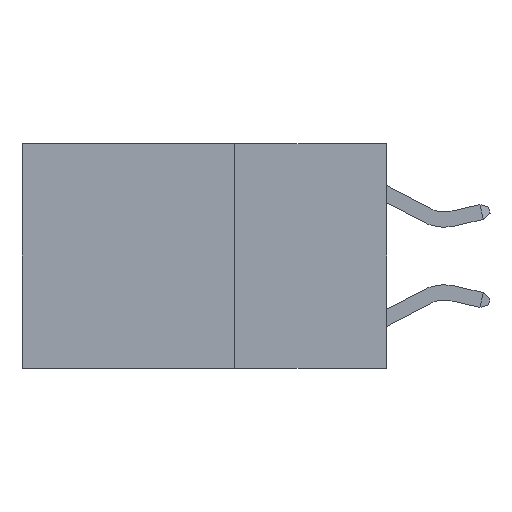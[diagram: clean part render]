
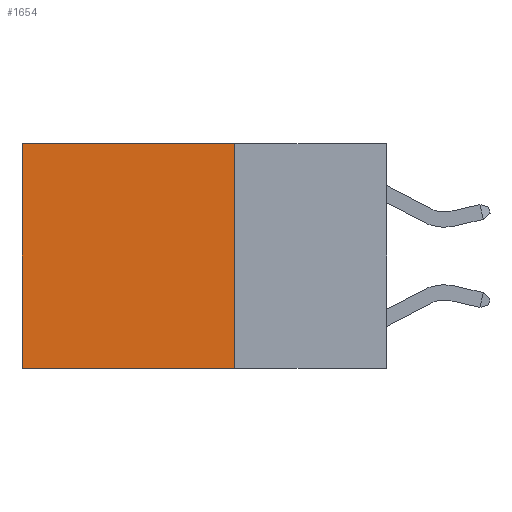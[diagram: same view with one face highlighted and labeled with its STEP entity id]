
A CAD part, left-side view. The second image highlights one B-rep face of the part: STEP entity #1654.
In plain terms, the highlighted planar face has unit normal (-1, 0, 0).
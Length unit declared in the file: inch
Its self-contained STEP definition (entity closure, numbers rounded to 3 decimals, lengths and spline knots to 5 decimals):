
#481 = VERTEX_POINT ( 'NONE', #1442 ) ;
#544 = EDGE_CURVE ( 'NONE', #481, #584, #4493, .T. ) ;
#584 = VERTEX_POINT ( 'NONE', #3467 ) ;
#688 = AXIS2_PLACEMENT_3D ( 'NONE', #9804, #9783, #9766 ) ;
#725 = CARTESIAN_POINT ( 'NONE',  ( 0.2625, 0.25, 0. ) ) ;
#829 = LINE ( 'NONE', #8729, #2874 ) ;
#1277 = CARTESIAN_POINT ( 'NONE',  ( 0.2625, 0.6, 0. ) ) ;
#1442 = CARTESIAN_POINT ( 'NONE',  ( 0.2625, 0.25, -0.37 ) ) ;
#1654 = ADVANCED_FACE ( 'NONE', ( #2584 ), #9794, .F. ) ;
#2584 = FACE_OUTER_BOUND ( 'NONE', #5169, .T. ) ;
#2874 = VECTOR ( 'NONE', #6541, 39.37008 ) ;
#3140 = LINE ( 'NONE', #725, #6587 ) ;
#3467 = CARTESIAN_POINT ( 'NONE',  ( 0.2625, 0.6, -0.37 ) ) ;
#3876 = LINE ( 'NONE', #1277, #5612 ) ;
#4258 = VECTOR ( 'NONE', #7129, 39.37008 ) ;
#4493 = LINE ( 'NONE', #5741, #4258 ) ;
#5169 = EDGE_LOOP ( 'NONE', ( #8312, #8377, #7961, #8511 ) ) ;
#5527 = EDGE_CURVE ( 'NONE', #7685, #481, #3140, .T. ) ;
#5612 = VECTOR ( 'NONE', #5980, 39.37008 ) ;
#5741 = CARTESIAN_POINT ( 'NONE',  ( 0.2625, 0.25, -0.37 ) ) ;
#5944 = EDGE_CURVE ( 'NONE', #6516, #584, #3876, .T. ) ;
#5980 = DIRECTION ( 'NONE',  ( 0., 0., -1. ) ) ;
#6516 = VERTEX_POINT ( 'NONE', #7720 ) ;
#6541 = DIRECTION ( 'NONE',  ( 0., 1., 0. ) ) ;
#6587 = VECTOR ( 'NONE', #7832, 39.37008 ) ;
#6941 = EDGE_CURVE ( 'NONE', #7685, #6516, #829, .T. ) ;
#7129 = DIRECTION ( 'NONE',  ( 0., 1., 0. ) ) ;
#7149 = CARTESIAN_POINT ( 'NONE',  ( 0.2625, 0.25, 0. ) ) ;
#7685 = VERTEX_POINT ( 'NONE', #7149 ) ;
#7720 = CARTESIAN_POINT ( 'NONE',  ( 0.2625, 0.6, 0. ) ) ;
#7832 = DIRECTION ( 'NONE',  ( 0., 0., -1. ) ) ;
#7961 = ORIENTED_EDGE ( 'NONE', *, *, #5527, .F. ) ;
#8312 = ORIENTED_EDGE ( 'NONE', *, *, #5944, .T. ) ;
#8377 = ORIENTED_EDGE ( 'NONE', *, *, #544, .F. ) ;
#8511 = ORIENTED_EDGE ( 'NONE', *, *, #6941, .T. ) ;
#8729 = CARTESIAN_POINT ( 'NONE',  ( 0.2625, 0.25, 0. ) ) ;
#9766 = DIRECTION ( 'NONE',  ( 0., 0., -1. ) ) ;
#9783 = DIRECTION ( 'NONE',  ( 1., 0., 0. ) ) ;
#9794 = PLANE ( 'NONE',  #688 ) ;
#9804 = CARTESIAN_POINT ( 'NONE',  ( 0.2625, 0.25, 0. ) ) ;
